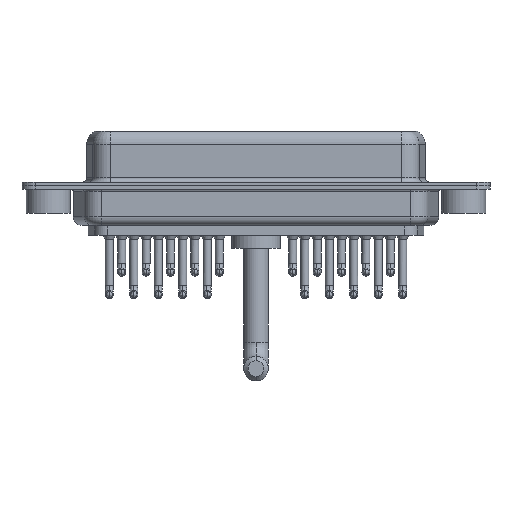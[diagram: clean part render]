
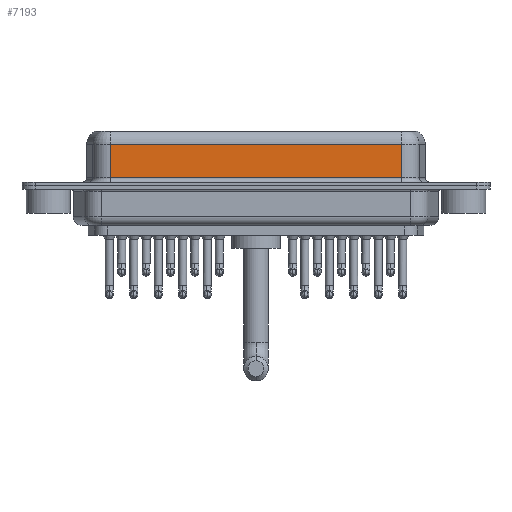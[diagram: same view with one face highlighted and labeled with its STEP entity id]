
A CAD part, front view. The second image highlights one B-rep face of the part: STEP entity #7193.
In plain terms, the highlighted planar face has unit normal (0, -1, 0).
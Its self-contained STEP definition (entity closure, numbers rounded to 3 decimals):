
#189 = ORIENTED_EDGE ( 'NONE', *, *, #20997, .F. ) ;
#502 = FACE_OUTER_BOUND ( 'NONE', #10430, .T. ) ;
#718 = CARTESIAN_POINT ( 'NONE',  ( 40.037, -3.95, 6.4 ) ) ;
#1029 = LINE ( 'NONE', #16436, #11958 ) ;
#1074 = VECTOR ( 'NONE', #11206, 1000. ) ;
#1965 = VERTEX_POINT ( 'NONE', #9638 ) ;
#2244 = ORIENTED_EDGE ( 'NONE', *, *, #21913, .T. ) ;
#2310 = ORIENTED_EDGE ( 'NONE', *, *, #18592, .T. ) ;
#5431 = CARTESIAN_POINT ( 'NONE',  ( 40.037, -3.95, 4.65 ) ) ;
#5927 = LINE ( 'NONE', #9373, #1074 ) ;
#6768 = CARTESIAN_POINT ( 'NONE',  ( 7.013, -3.95, 4.65 ) ) ;
#7193 = ADVANCED_FACE ( 'NONE', ( #502 ), #16451, .F. ) ;
#7812 = CARTESIAN_POINT ( 'NONE',  ( 40.037, -3.95, 4.65 ) ) ;
#8180 = DIRECTION ( 'NONE',  ( 1., 0., 0. ) ) ;
#8754 = CARTESIAN_POINT ( 'NONE',  ( 7.013, -3.95, 0.9 ) ) ;
#8846 = VERTEX_POINT ( 'NONE', #6768 ) ;
#8874 = CARTESIAN_POINT ( 'NONE',  ( 40.037, -3.95, 6.4 ) ) ;
#9223 = ORIENTED_EDGE ( 'NONE', *, *, #17602, .T. ) ;
#9373 = CARTESIAN_POINT ( 'NONE',  ( 7.013, -3.95, 6.4 ) ) ;
#9626 = AXIS2_PLACEMENT_3D ( 'NONE', #718, #14739, #10847 ) ;
#9638 = CARTESIAN_POINT ( 'NONE',  ( 40.037, -3.95, 0.9 ) ) ;
#10430 = EDGE_LOOP ( 'NONE', ( #189, #2310, #2244, #9223 ) ) ;
#10818 = LINE ( 'NONE', #8874, #19393 ) ;
#10847 = DIRECTION ( 'NONE',  ( 0., 0., 1. ) ) ;
#11206 = DIRECTION ( 'NONE',  ( 0., 0., -1. ) ) ;
#11958 = VECTOR ( 'NONE', #8180, 1000. ) ;
#13447 = VECTOR ( 'NONE', #15632, 1000. ) ;
#14739 = DIRECTION ( 'NONE',  ( 0., 1., 0. ) ) ;
#15571 = VERTEX_POINT ( 'NONE', #7812 ) ;
#15632 = DIRECTION ( 'NONE',  ( -1., 0., 0. ) ) ;
#16436 = CARTESIAN_POINT ( 'NONE',  ( 40.037, -3.95, 0.9 ) ) ;
#16451 = PLANE ( 'NONE',  #9626 ) ;
#17252 = LINE ( 'NONE', #5431, #13447 ) ;
#17602 = EDGE_CURVE ( 'NONE', #21092, #1965, #1029, .T. ) ;
#18592 = EDGE_CURVE ( 'NONE', #15571, #8846, #17252, .T. ) ;
#19393 = VECTOR ( 'NONE', #21355, 1000. ) ;
#20997 = EDGE_CURVE ( 'NONE', #15571, #1965, #10818, .T. ) ;
#21092 = VERTEX_POINT ( 'NONE', #8754 ) ;
#21355 = DIRECTION ( 'NONE',  ( 0., 0., -1. ) ) ;
#21913 = EDGE_CURVE ( 'NONE', #8846, #21092, #5927, .T. ) ;
